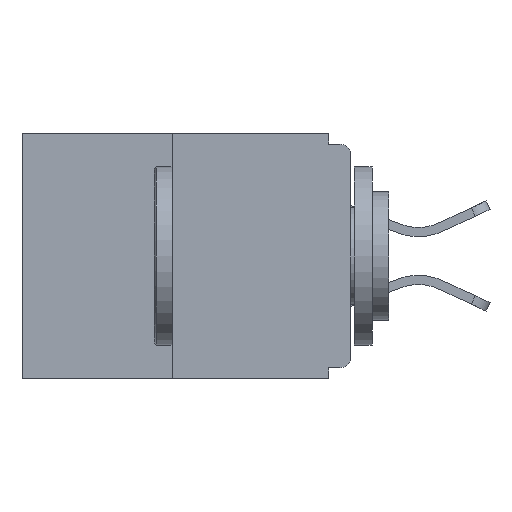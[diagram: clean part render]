
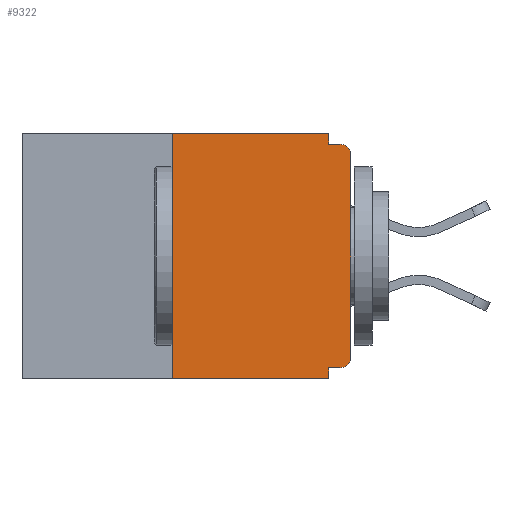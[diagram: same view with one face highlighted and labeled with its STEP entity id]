
A CAD part, left-side view. The second image highlights one B-rep face of the part: STEP entity #9322.
In plain terms, the highlighted planar face has unit normal (-1, 0, 0).
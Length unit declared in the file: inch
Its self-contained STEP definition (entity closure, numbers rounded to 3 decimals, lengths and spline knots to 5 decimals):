
#18 = VERTEX_POINT ( 'NONE', #12124 ) ;
#180 = VECTOR ( 'NONE', #4815, 39.37008 ) ;
#280 = DIRECTION ( 'NONE',  ( 0., 0., -1. ) ) ;
#281 = EDGE_CURVE ( 'NONE', #562, #6743, #3030, .T. ) ;
#450 = CARTESIAN_POINT ( 'NONE',  ( 0., 0.015, -0.015 ) ) ;
#459 = CARTESIAN_POINT ( 'NONE',  ( 0., 0.25, 0. ) ) ;
#496 = DIRECTION ( 'NONE',  ( 0., 0., 1. ) ) ;
#562 = VERTEX_POINT ( 'NONE', #11576 ) ;
#923 = DIRECTION ( 'NONE',  ( 0., 0., 1. ) ) ;
#1063 = VECTOR ( 'NONE', #2924, 39.37008 ) ;
#1066 = EDGE_CURVE ( 'NONE', #10689, #1112, #8024, .T. ) ;
#1112 = VERTEX_POINT ( 'NONE', #450 ) ;
#1328 = VERTEX_POINT ( 'NONE', #9596 ) ;
#1375 = ORIENTED_EDGE ( 'NONE', *, *, #3583, .F. ) ;
#1522 = LINE ( 'NONE', #2768, #1944 ) ;
#1530 = LINE ( 'NONE', #459, #9480 ) ;
#1639 = AXIS2_PLACEMENT_3D ( 'NONE', #3949, #11548, #280 ) ;
#1854 = DIRECTION ( 'NONE',  ( 0., 0., -1. ) ) ;
#1944 = VECTOR ( 'NONE', #1854, 39.37008 ) ;
#2537 = CARTESIAN_POINT ( 'NONE',  ( 0., 0., -0.313 ) ) ;
#2692 = LINE ( 'NONE', #9498, #180 ) ;
#2768 = CARTESIAN_POINT ( 'NONE',  ( 0., 0.031, -0.343 ) ) ;
#2800 = ORIENTED_EDGE ( 'NONE', *, *, #281, .T. ) ;
#2924 = DIRECTION ( 'NONE',  ( 0., 0., -1. ) ) ;
#3030 = CIRCLE ( 'NONE', #10677, 0.015 ) ;
#3103 = EDGE_CURVE ( 'NONE', #1328, #10689, #7239, .T. ) ;
#3256 = LINE ( 'NONE', #5729, #4582 ) ;
#3455 = VERTEX_POINT ( 'NONE', #9284 ) ;
#3583 = EDGE_CURVE ( 'NONE', #562, #18, #3256, .T. ) ;
#3852 = ORIENTED_EDGE ( 'NONE', *, *, #7414, .T. ) ;
#3949 = CARTESIAN_POINT ( 'NONE',  ( 0., 0.015, -0.03 ) ) ;
#4243 = ORIENTED_EDGE ( 'NONE', *, *, #10988, .F. ) ;
#4354 = VERTEX_POINT ( 'NONE', #11594 ) ;
#4582 = VECTOR ( 'NONE', #8563, 39.37008 ) ;
#4815 = DIRECTION ( 'NONE',  ( 0., -1., 0. ) ) ;
#5036 = DIRECTION ( 'NONE',  ( -1., 0., 0. ) ) ;
#5087 = CARTESIAN_POINT ( 'NONE',  ( 0., 0.46, 0. ) ) ;
#5548 = ORIENTED_EDGE ( 'NONE', *, *, #10873, .T. ) ;
#5575 = LINE ( 'NONE', #8231, #8813 ) ;
#5729 = CARTESIAN_POINT ( 'NONE',  ( 0., 0., -0.328 ) ) ;
#5893 = EDGE_CURVE ( 'NONE', #6743, #3455, #8186, .T. ) ;
#5920 = AXIS2_PLACEMENT_3D ( 'NONE', #5087, #7860, #5990 ) ;
#5966 = ORIENTED_EDGE ( 'NONE', *, *, #8214, .F. ) ;
#5990 = DIRECTION ( 'NONE',  ( 0., 0., -1. ) ) ;
#6085 = DIRECTION ( 'NONE',  ( 0., -1., 0. ) ) ;
#6298 = VERTEX_POINT ( 'NONE', #11056 ) ;
#6471 = DIRECTION ( 'NONE',  ( 0., -1., 0. ) ) ;
#6522 = CARTESIAN_POINT ( 'NONE',  ( 0., 0., -0.015 ) ) ;
#6743 = VERTEX_POINT ( 'NONE', #2537 ) ;
#7084 = EDGE_LOOP ( 'NONE', ( #5966, #9855, #5548, #4243, #1375, #2800, #9510, #3852, #8413, #7364 ) ) ;
#7239 = LINE ( 'NONE', #11113, #1063 ) ;
#7364 = ORIENTED_EDGE ( 'NONE', *, *, #3103, .F. ) ;
#7414 = EDGE_CURVE ( 'NONE', #3455, #1112, #9256, .T. ) ;
#7860 = DIRECTION ( 'NONE',  ( 1., 0., 0. ) ) ;
#8024 = LINE ( 'NONE', #6522, #8613 ) ;
#8186 = LINE ( 'NONE', #10403, #9105 ) ;
#8214 = EDGE_CURVE ( 'NONE', #11010, #1328, #5575, .T. ) ;
#8231 = CARTESIAN_POINT ( 'NONE',  ( 0., 0.46, 0. ) ) ;
#8413 = ORIENTED_EDGE ( 'NONE', *, *, #1066, .F. ) ;
#8563 = DIRECTION ( 'NONE',  ( 0., 1., 0. ) ) ;
#8613 = VECTOR ( 'NONE', #6085, 39.37008 ) ;
#8813 = VECTOR ( 'NONE', #6471, 39.37008 ) ;
#8876 = PLANE ( 'NONE',  #5920 ) ;
#8911 = CARTESIAN_POINT ( 'NONE',  ( 0., 0.25, 0. ) ) ;
#9105 = VECTOR ( 'NONE', #923, 39.37008 ) ;
#9256 = CIRCLE ( 'NONE', #1639, 0.015 ) ;
#9284 = CARTESIAN_POINT ( 'NONE',  ( 0., 0., -0.03 ) ) ;
#9322 = ADVANCED_FACE ( 'NONE', ( #11405 ), #8876, .F. ) ;
#9480 = VECTOR ( 'NONE', #496, 39.37008 ) ;
#9498 = CARTESIAN_POINT ( 'NONE',  ( 0., 0.46, -0.343 ) ) ;
#9510 = ORIENTED_EDGE ( 'NONE', *, *, #5893, .T. ) ;
#9596 = CARTESIAN_POINT ( 'NONE',  ( 0., 0.031, 0. ) ) ;
#9855 = ORIENTED_EDGE ( 'NONE', *, *, #10503, .F. ) ;
#10403 = CARTESIAN_POINT ( 'NONE',  ( 0., 0., 0. ) ) ;
#10503 = EDGE_CURVE ( 'NONE', #6298, #11010, #1530, .T. ) ;
#10639 = CARTESIAN_POINT ( 'NONE',  ( 0., 0.015, -0.313 ) ) ;
#10677 = AXIS2_PLACEMENT_3D ( 'NONE', #10639, #5036, #11597 ) ;
#10689 = VERTEX_POINT ( 'NONE', #10698 ) ;
#10698 = CARTESIAN_POINT ( 'NONE',  ( 0., 0.031, -0.015 ) ) ;
#10873 = EDGE_CURVE ( 'NONE', #6298, #4354, #2692, .T. ) ;
#10988 = EDGE_CURVE ( 'NONE', #18, #4354, #1522, .T. ) ;
#11010 = VERTEX_POINT ( 'NONE', #8911 ) ;
#11056 = CARTESIAN_POINT ( 'NONE',  ( 0., 0.25, -0.343 ) ) ;
#11113 = CARTESIAN_POINT ( 'NONE',  ( 0., 0.031, 0. ) ) ;
#11405 = FACE_OUTER_BOUND ( 'NONE', #7084, .T. ) ;
#11548 = DIRECTION ( 'NONE',  ( -1., 0., 0. ) ) ;
#11576 = CARTESIAN_POINT ( 'NONE',  ( 0., 0.015, -0.328 ) ) ;
#11594 = CARTESIAN_POINT ( 'NONE',  ( 0., 0.031, -0.343 ) ) ;
#11597 = DIRECTION ( 'NONE',  ( 0., 0., -1. ) ) ;
#12124 = CARTESIAN_POINT ( 'NONE',  ( 0., 0.031, -0.328 ) ) ;
